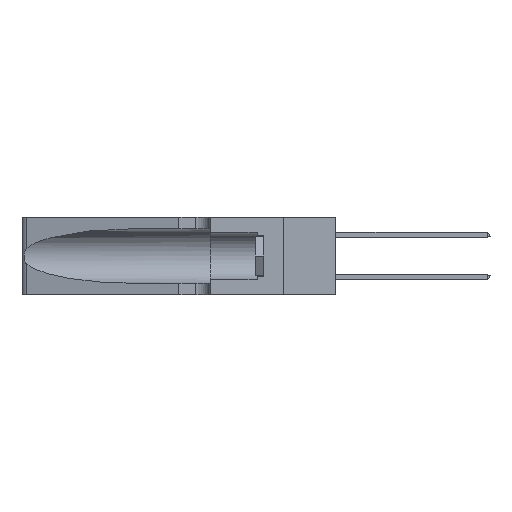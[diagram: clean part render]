
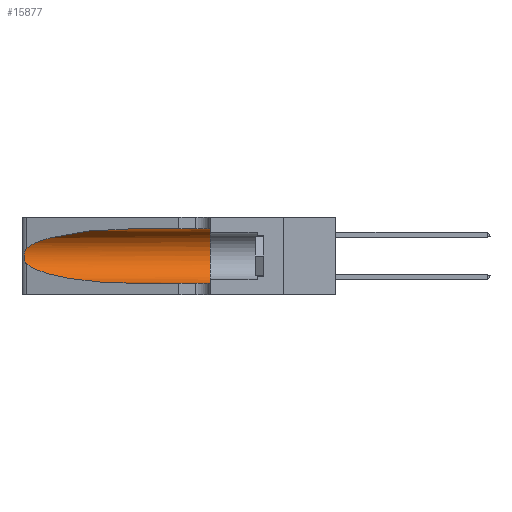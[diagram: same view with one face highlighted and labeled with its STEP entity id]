
A CAD part, left-side view. The second image highlights one B-rep face of the part: STEP entity #15877.
In plain terms, the highlighted cylindrical face has radius 3.308 mm (diameter 6.617 mm), a partial arc.
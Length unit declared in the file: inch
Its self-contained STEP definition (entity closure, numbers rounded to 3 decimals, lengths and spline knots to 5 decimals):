
#314 = LINE ( 'NONE', #6491, #24982 ) ;
#715 = VERTEX_POINT ( 'NONE', #11263 ) ;
#1433 = VERTEX_POINT ( 'NONE', #9363 ) ;
#1582 = CARTESIAN_POINT ( 'NONE',  ( 0.25555, 1.22994, 0.2215 ) ) ;
#1695 = CARTESIAN_POINT ( 'NONE',  ( 0.25639, 1.23186, 0.15144 ) ) ;
#3395 = CARTESIAN_POINT ( 'NONE',  ( 0.1305, 0.35, 0.185 ) ) ;
#4230 = CARTESIAN_POINT ( 'NONE',  ( 0.25487, 1.22718, 0.14631 ) ) ;
#4388 = VERTEX_POINT ( 'NONE', #21864 ) ;
#4843 = VECTOR ( 'NONE', #16443, 39.37008 ) ;
#5249 = CYLINDRICAL_SURFACE ( 'NONE', #23675, 0.13025 ) ;
#5917 = DIRECTION ( 'NONE',  ( 0., 0., 1. ) ) ;
#6491 = CARTESIAN_POINT ( 'NONE',  ( 0.1305, 1.61858, 0.05475 ) ) ;
#6500 =( BOUNDED_CURVE ( )  B_SPLINE_CURVE ( 3, ( #17306, #19737, #27009, #12505 ),
 .UNSPECIFIED., .F., .T. ) 
 B_SPLINE_CURVE_WITH_KNOTS ( ( 4, 4 ),
 ( 3.44316, 4.71239 ),
 .UNSPECIFIED. ) 
 CURVE ( )  GEOMETRIC_REPRESENTATION_ITEM ( )  RATIONAL_B_SPLINE_CURVE ( ( 1., 0.87, 0.87, 1. ) ) 
 REPRESENTATION_ITEM ( '' )  );
#6515 = CARTESIAN_POINT ( 'NONE',  ( 0.1305, 1.61858, 0.31525 ) ) ;
#6643 = CARTESIAN_POINT ( 'NONE',  ( 0.25639, 1.23184, 0.21858 ) ) ;
#7672 = CARTESIAN_POINT ( 'NONE',  ( 0.1305, 0.35, 0.31525 ) ) ;
#8362 = VERTEX_POINT ( 'NONE', #25446 ) ;
#9153 = CARTESIAN_POINT ( 'NONE',  ( 0.25854, 1.2359, 0.20912 ) ) ;
#9357 = CIRCLE ( 'NONE', #30510, 0.13025 ) ;
#9363 = CARTESIAN_POINT ( 'NONE',  ( 0.1305, 0.72297, 0.31525 ) ) ;
#9741 = CARTESIAN_POINT ( 'NONE',  ( 0.25487, 1.22718, 0.22369 ) ) ;
#9826 = ORIENTED_EDGE ( 'NONE', *, *, #14356, .T. ) ;
#11263 = CARTESIAN_POINT ( 'NONE',  ( 0.1305, 0.35, 0.05475 ) ) ;
#11338 = CARTESIAN_POINT ( 'NONE',  ( 0.2373, 1.15595, 0.28018 ) ) ;
#11669 = CARTESIAN_POINT ( 'NONE',  ( 0.26075, 1.23896, 0.19203 ) ) ;
#12290 =( BOUNDED_CURVE ( )  B_SPLINE_CURVE ( 3, ( #23468, #25866, #11338, #28278 ),
 .UNSPECIFIED., .F., .F. ) 
 B_SPLINE_CURVE_WITH_KNOTS ( ( 4, 4 ),
 ( 1.5708, 2.84003 ),
 .UNSPECIFIED. ) 
 CURVE ( )  GEOMETRIC_REPRESENTATION_ITEM ( )  RATIONAL_B_SPLINE_CURVE ( ( 1., 0.87, 0.87, 1. ) ) 
 REPRESENTATION_ITEM ( '' )  );
#12505 = CARTESIAN_POINT ( 'NONE',  ( 0.1305, 0.72297, 0.05475 ) ) ;
#12947 = ORIENTED_EDGE ( 'NONE', *, *, #26427, .F. ) ;
#13054 = ORIENTED_EDGE ( 'NONE', *, *, #14073, .T. ) ;
#13074 = VERTEX_POINT ( 'NONE', #9741 ) ;
#13540 = CARTESIAN_POINT ( 'NONE',  ( 0.1305, 1.61858, 0.185 ) ) ;
#14073 = EDGE_CURVE ( 'NONE', #1433, #13074, #12290, .T. ) ;
#14139 = CARTESIAN_POINT ( 'NONE',  ( 0.26017, 1.23833, 0.17102 ) ) ;
#14356 = EDGE_CURVE ( 'NONE', #4388, #8362, #6500, .T. ) ;
#14716 = EDGE_CURVE ( 'NONE', #8362, #715, #314, .T. ) ;
#15877 = ADVANCED_FACE ( 'NONE', ( #24784 ), #5249, .F. ) ;
#16256 = EDGE_LOOP ( 'NONE', ( #13054, #29757, #9826, #20075, #12947, #22581 ) ) ;
#16443 = DIRECTION ( 'NONE',  ( 0., -1., 0. ) ) ;
#16580 = CARTESIAN_POINT ( 'NONE',  ( 0.25789, 1.23486, 0.15765 ) ) ;
#17306 = CARTESIAN_POINT ( 'NONE',  ( 0.25487, 1.22718, 0.14631 ) ) ;
#18922 = CARTESIAN_POINT ( 'NONE',  ( 0.25487, 1.22718, 0.22369 ) ) ;
#19025 = CARTESIAN_POINT ( 'NONE',  ( 0.25555, 1.22993, 0.14849 ) ) ;
#19737 = CARTESIAN_POINT ( 'NONE',  ( 0.2373, 1.15595, 0.08982 ) ) ;
#20075 = ORIENTED_EDGE ( 'NONE', *, *, #14716, .T. ) ;
#20651 = DIRECTION ( 'NONE',  ( 0., 1., 0. ) ) ;
#21864 = CARTESIAN_POINT ( 'NONE',  ( 0.25487, 1.22718, 0.14631 ) ) ;
#22581 = ORIENTED_EDGE ( 'NONE', *, *, #24089, .F. ) ;
#23043 = VERTEX_POINT ( 'NONE', #7672 ) ;
#23468 = CARTESIAN_POINT ( 'NONE',  ( 0.1305, 0.72297, 0.31525 ) ) ;
#23675 = AXIS2_PLACEMENT_3D ( 'NONE', #13540, #30404, #25596 ) ;
#23782 = CARTESIAN_POINT ( 'NONE',  ( 0.25787, 1.23484, 0.2124 ) ) ;
#24089 = EDGE_CURVE ( 'NONE', #1433, #23043, #30021, .T. ) ;
#24784 = FACE_OUTER_BOUND ( 'NONE', #16256, .T. ) ;
#24982 = VECTOR ( 'NONE', #26042, 39.37008 ) ;
#25446 = CARTESIAN_POINT ( 'NONE',  ( 0.1305, 0.72297, 0.05475 ) ) ;
#25596 = DIRECTION ( 'NONE',  ( 0., 0., -1. ) ) ;
#25866 = CARTESIAN_POINT ( 'NONE',  ( 0.18966, 0.96281, 0.31525 ) ) ;
#26042 = DIRECTION ( 'NONE',  ( 0., -1., 0. ) ) ;
#26183 = CARTESIAN_POINT ( 'NONE',  ( 0.26018, 1.23835, 0.19895 ) ) ;
#26427 = EDGE_CURVE ( 'NONE', #23043, #715, #9357, .T. ) ;
#27009 = CARTESIAN_POINT ( 'NONE',  ( 0.18966, 0.96281, 0.05475 ) ) ;
#28209 = EDGE_CURVE ( 'NONE', #13074, #4388, #30116, .T. ) ;
#28278 = CARTESIAN_POINT ( 'NONE',  ( 0.25487, 1.22718, 0.22369 ) ) ;
#28596 = CARTESIAN_POINT ( 'NONE',  ( 0.26075, 1.23896, 0.178 ) ) ;
#29757 = ORIENTED_EDGE ( 'NONE', *, *, #28209, .T. ) ;
#30021 = LINE ( 'NONE', #6515, #4843 ) ;
#30116 = B_SPLINE_CURVE_WITH_KNOTS ( 'NONE', 3,
 ( #18922, #1582, #6643, #23782, #9153, #26183, #11669, #28596, #14139, #30975, #16580, #1695, #19025, #4230 ),
 .UNSPECIFIED., .F., .F.,
 ( 4, 2, 2, 2, 2, 2, 4 ),
 ( 0., 0.00027, 0.00053, 0.00107, 0.0016, 0.00187, 0.00214 ),
 .UNSPECIFIED. ) ;
#30404 = DIRECTION ( 'NONE',  ( 0., -1., 0. ) ) ;
#30510 = AXIS2_PLACEMENT_3D ( 'NONE', #3395, #20651, #5917 ) ;
#30975 = CARTESIAN_POINT ( 'NONE',  ( 0.25856, 1.23593, 0.16098 ) ) ;
